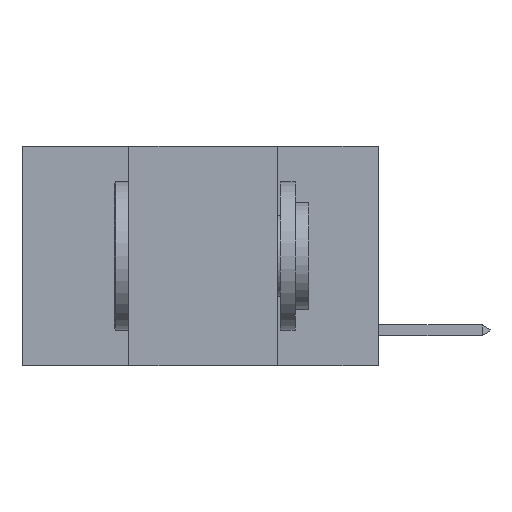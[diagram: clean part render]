
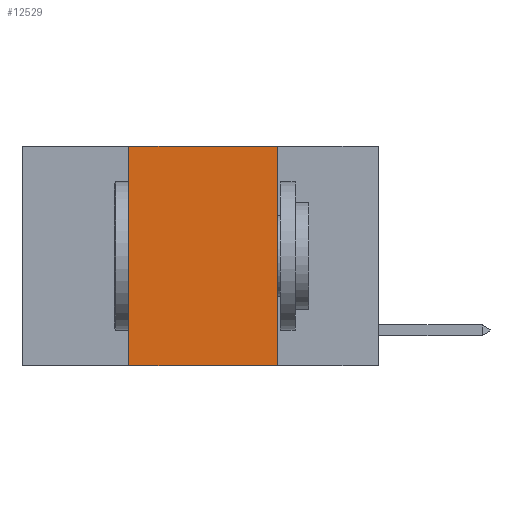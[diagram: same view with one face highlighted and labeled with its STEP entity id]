
A CAD part, left-side view. The second image highlights one B-rep face of the part: STEP entity #12529.
In plain terms, the highlighted planar face has unit normal (-1, 0, 0).
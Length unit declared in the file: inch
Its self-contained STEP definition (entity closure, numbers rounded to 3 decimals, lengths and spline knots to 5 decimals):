
#272 = LINE ( 'NONE', #11673, #9936 ) ;
#334 = DIRECTION ( 'NONE',  ( 0., 0., -1. ) ) ;
#1420 = DIRECTION ( 'NONE',  ( 0., 0., 1. ) ) ;
#1424 = CARTESIAN_POINT ( 'NONE',  ( 0., 0.17, 0. ) ) ;
#1507 = DIRECTION ( 'NONE',  ( 0., 0., -1. ) ) ;
#1783 = FACE_OUTER_BOUND ( 'NONE', #26441, .T. ) ;
#3156 = EDGE_CURVE ( 'NONE', #21048, #16071, #23577, .T. ) ;
#4513 = ORIENTED_EDGE ( 'NONE', *, *, #3156, .F. ) ;
#7297 = VECTOR ( 'NONE', #18902, 39.37008 ) ;
#8043 = VECTOR ( 'NONE', #334, 39.37008 ) ;
#9140 = VECTOR ( 'NONE', #15191, 39.37008 ) ;
#9936 = VECTOR ( 'NONE', #1420, 39.37008 ) ;
#10421 = LINE ( 'NONE', #15285, #9140 ) ;
#11270 = CARTESIAN_POINT ( 'NONE',  ( 0., 0.42, 0. ) ) ;
#11539 = VERTEX_POINT ( 'NONE', #26025 ) ;
#11673 = CARTESIAN_POINT ( 'NONE',  ( 0., 0.42, 0. ) ) ;
#11752 = PLANE ( 'NONE',  #26476 ) ;
#12529 = ADVANCED_FACE ( 'NONE', ( #1783 ), #11752, .F. ) ;
#13194 = VERTEX_POINT ( 'NONE', #13903 ) ;
#13841 = DIRECTION ( 'NONE',  ( 1., 0., 0. ) ) ;
#13903 = CARTESIAN_POINT ( 'NONE',  ( 0., 0.42, -0.37 ) ) ;
#14722 = CARTESIAN_POINT ( 'NONE',  ( 0., 0.17, 0. ) ) ;
#14791 = CARTESIAN_POINT ( 'NONE',  ( 0., 0.6, 0. ) ) ;
#15191 = DIRECTION ( 'NONE',  ( 0., -1., 0. ) ) ;
#15285 = CARTESIAN_POINT ( 'NONE',  ( 0., 0.6, -0.37 ) ) ;
#16071 = VERTEX_POINT ( 'NONE', #1424 ) ;
#18902 = DIRECTION ( 'NONE',  ( 0., -1., 0. ) ) ;
#20214 = ORIENTED_EDGE ( 'NONE', *, *, #22168, .F. ) ;
#21048 = VERTEX_POINT ( 'NONE', #11270 ) ;
#22168 = EDGE_CURVE ( 'NONE', #16071, #11539, #24325, .T. ) ;
#22742 = ORIENTED_EDGE ( 'NONE', *, *, #26253, .F. ) ;
#23541 = EDGE_CURVE ( 'NONE', #13194, #11539, #10421, .T. ) ;
#23577 = LINE ( 'NONE', #14791, #7297 ) ;
#24325 = LINE ( 'NONE', #14722, #8043 ) ;
#24684 = ORIENTED_EDGE ( 'NONE', *, *, #23541, .T. ) ;
#25995 = CARTESIAN_POINT ( 'NONE',  ( 0., 0.6, 0. ) ) ;
#26025 = CARTESIAN_POINT ( 'NONE',  ( 0., 0.17, -0.37 ) ) ;
#26253 = EDGE_CURVE ( 'NONE', #13194, #21048, #272, .T. ) ;
#26441 = EDGE_LOOP ( 'NONE', ( #20214, #4513, #22742, #24684 ) ) ;
#26476 = AXIS2_PLACEMENT_3D ( 'NONE', #25995, #13841, #1507 ) ;
